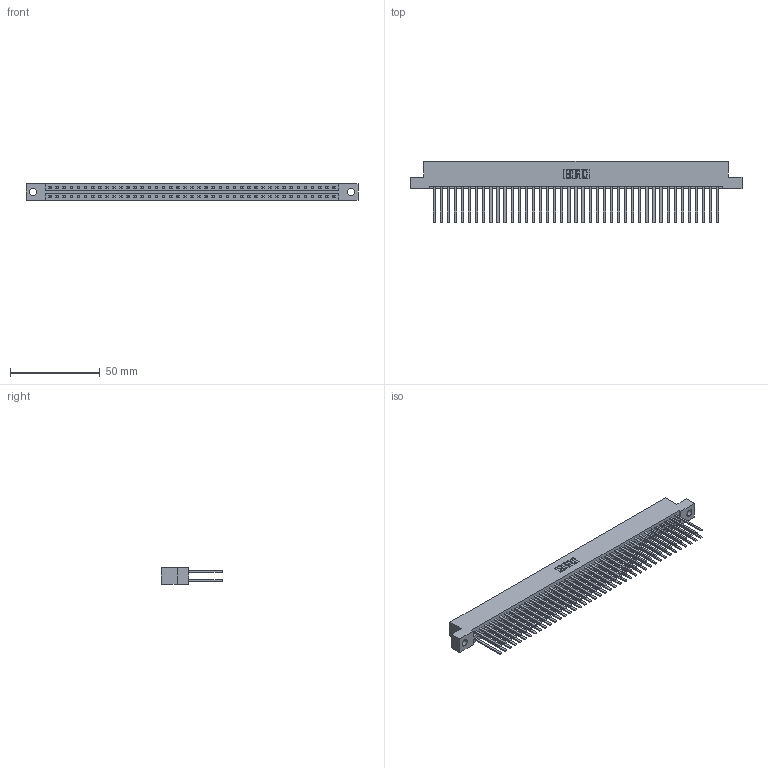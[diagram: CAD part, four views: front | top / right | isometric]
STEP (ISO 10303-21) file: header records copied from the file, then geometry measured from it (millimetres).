
FILE_DESCRIPTION (( 'STEP AP203' ), '1' );
FILE_NAME ('387-082-544-204.STEP', '2018-09-23T20:29:49', ( '' ), ( '' ), 'SwSTEP 2.0', 'SolidWorks 2016', '' );
FILE_SCHEMA (( 'CONFIG_CONTROL_DESIGN' ));
Length unit declared in the file: inch
Products named in the file (3): 387-082-544-204; 337 Part_Flush Mounting Lugs - 0.156 Dia-TH; 345-292-001_345-293-144
Assembly tree (83 placements, depth 2):
  387-082-544-204
    337 Part_Flush Mounting Lugs - 0.156 Dia-TH
    345-292-001_345-293-144  x82
Bounding box: 185.47 x 34.3 x 9.4 mm (x, y, z)
Volume: 20594.7 mm3; surface area: 26825.1 mm2
Topology: 83 solids, 83 shells, 4050 faces, 12037 edges, 7914 vertices
Faces by surface type: plane 2858, cylinder 1192
Entity records: 31737 total; most frequent: CARTESIAN_POINT 5346, ORIENTED_EDGE 5282, DIRECTION 4545, EDGE_CURVE 2641, VECTOR 2517, LINE 2517, VERTEX_POINT 1758, AXIS2_PLACEMENT_3D 1014
